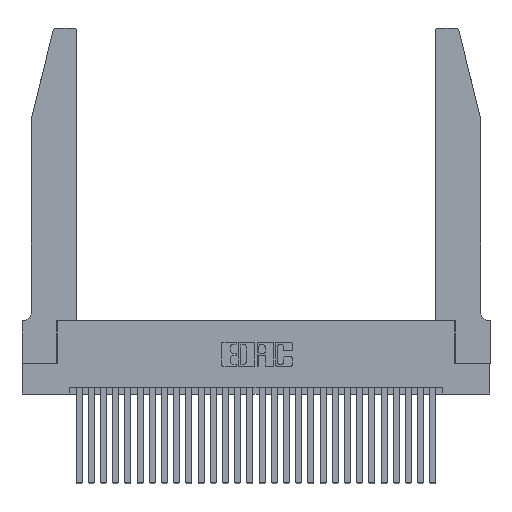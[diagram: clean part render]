
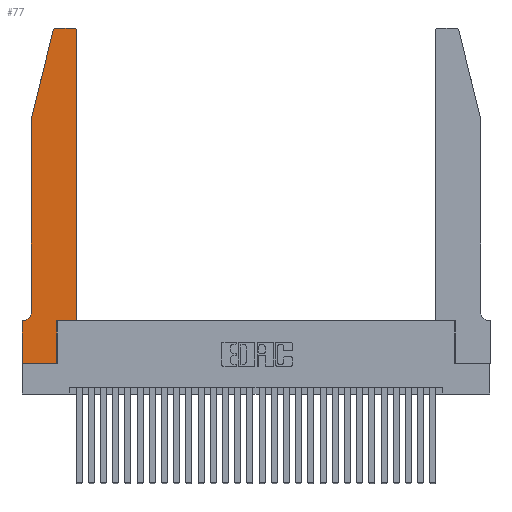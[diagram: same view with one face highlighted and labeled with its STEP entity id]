
A CAD part, top view. The second image highlights one B-rep face of the part: STEP entity #77.
In plain terms, the highlighted planar face has unit normal (0, 0, 1).
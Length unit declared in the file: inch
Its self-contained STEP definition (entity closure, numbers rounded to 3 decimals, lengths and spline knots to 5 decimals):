
#77 = ADVANCED_FACE ( 'NONE', ( #26338 ), #5911, .T. ) ;
#261 = DIRECTION ( 'NONE',  ( -0.239, -0.971, 0. ) ) ;
#552 = DIRECTION ( 'NONE',  ( -1., 0., 0. ) ) ;
#562 = ORIENTED_EDGE ( 'NONE', *, *, #4108, .T. ) ;
#1627 = DIRECTION ( 'NONE',  ( -1., 0., 0. ) ) ;
#1837 = ORIENTED_EDGE ( 'NONE', *, *, #16218, .T. ) ;
#2199 = VECTOR ( 'NONE', #18765, 39.37008 ) ;
#2435 = CARTESIAN_POINT ( 'NONE',  ( 0.284, 2.75, 0.37 ) ) ;
#3099 = DIRECTION ( 'NONE',  ( 0., -1., 0. ) ) ;
#3927 = CARTESIAN_POINT ( 'NONE',  ( 0.4205, 2.75, 0.37 ) ) ;
#4108 = EDGE_CURVE ( 'NONE', #5918, #16222, #10829, .T. ) ;
#5079 = EDGE_CURVE ( 'NONE', #28512, #18662, #29713, .T. ) ;
#5210 = ORIENTED_EDGE ( 'NONE', *, *, #26392, .T. ) ;
#5576 = VECTOR ( 'NONE', #8357, 39.37008 ) ;
#5631 = LINE ( 'NONE', #8975, #16499 ) ;
#5864 = DIRECTION ( 'NONE',  ( 0., 1., 0. ) ) ;
#5896 = VECTOR ( 'NONE', #9201, 39.37008 ) ;
#5911 = PLANE ( 'NONE',  #17791 ) ;
#5918 = VERTEX_POINT ( 'NONE', #26339 ) ;
#6234 = AXIS2_PLACEMENT_3D ( 'NONE', #11985, #27844, #14289 ) ;
#7351 = LINE ( 'NONE', #25167, #5896 ) ;
#8357 = DIRECTION ( 'NONE',  ( 1., 0., 0. ) ) ;
#8621 = EDGE_CURVE ( 'NONE', #22526, #9261, #5631, .T. ) ;
#8630 = CARTESIAN_POINT ( 'NONE',  ( 0., 0.35, 0.37 ) ) ;
#8869 = LINE ( 'NONE', #22281, #13567 ) ;
#8975 = CARTESIAN_POINT ( 'NONE',  ( 0., 0., 0.37 ) ) ;
#9042 = CARTESIAN_POINT ( 'NONE',  ( 0.2865, 0., 0.37 ) ) ;
#9201 = DIRECTION ( 'NONE',  ( 0., -1., 0. ) ) ;
#9261 = VERTEX_POINT ( 'NONE', #9042 ) ;
#9852 = ORIENTED_EDGE ( 'NONE', *, *, #10939, .T. ) ;
#9996 = CARTESIAN_POINT ( 'NONE',  ( 0.2605, 2.75, 0.37 ) ) ;
#10221 = VERTEX_POINT ( 'NONE', #15448 ) ;
#10367 = DIRECTION ( 'NONE',  ( 0., 0., 1. ) ) ;
#10577 = CARTESIAN_POINT ( 'NONE',  ( 0.4505, 0.35, 0.37 ) ) ;
#10829 = CIRCLE ( 'NONE', #6234, 0.03 ) ;
#10939 = EDGE_CURVE ( 'NONE', #20182, #22526, #7351, .T. ) ;
#11081 = EDGE_CURVE ( 'NONE', #12643, #5918, #14593, .T. ) ;
#11454 = VECTOR ( 'NONE', #5864, 39.37008 ) ;
#11659 = CARTESIAN_POINT ( 'NONE',  ( 0., 0., 0.37 ) ) ;
#11985 = CARTESIAN_POINT ( 'NONE',  ( 0.4205, 2.72, 0.37 ) ) ;
#12000 = CIRCLE ( 'NONE', #26807, 0.07 ) ;
#12643 = VERTEX_POINT ( 'NONE', #28993 ) ;
#12751 = ORIENTED_EDGE ( 'NONE', *, *, #15363, .T. ) ;
#13154 = CARTESIAN_POINT ( 'NONE',  ( 0.25487, 2.72718, 0.37 ) ) ;
#13567 = VECTOR ( 'NONE', #29037, 39.37008 ) ;
#14289 = DIRECTION ( 'NONE',  ( 1., 0., 0. ) ) ;
#14382 = CARTESIAN_POINT ( 'NONE',  ( 0.0755, 2., 0.37 ) ) ;
#14593 = LINE ( 'NONE', #16482, #2199 ) ;
#14709 = VECTOR ( 'NONE', #3099, 39.37008 ) ;
#15054 = ORIENTED_EDGE ( 'NONE', *, *, #11081, .T. ) ;
#15118 = CARTESIAN_POINT ( 'NONE',  ( 0.0755, 2., 0.37 ) ) ;
#15363 = EDGE_CURVE ( 'NONE', #16222, #23234, #18998, .T. ) ;
#15448 = CARTESIAN_POINT ( 'NONE',  ( 0.2865, 0.35, 0.37 ) ) ;
#15557 = DIRECTION ( 'NONE',  ( 0., 0., -1. ) ) ;
#16218 = EDGE_CURVE ( 'NONE', #18629, #20182, #8869, .T. ) ;
#16222 = VERTEX_POINT ( 'NONE', #3927 ) ;
#16482 = CARTESIAN_POINT ( 'NONE',  ( 0.4505, 0.35, 0.37 ) ) ;
#16499 = VECTOR ( 'NONE', #29437, 39.37008 ) ;
#16911 = ORIENTED_EDGE ( 'NONE', *, *, #19926, .T. ) ;
#17079 = VECTOR ( 'NONE', #261, 39.37008 ) ;
#17348 = CARTESIAN_POINT ( 'NONE',  ( 0.0055, 0.35, 0.37 ) ) ;
#17791 = AXIS2_PLACEMENT_3D ( 'NONE', #23497, #18524, #18530 ) ;
#17871 = LINE ( 'NONE', #10577, #5576 ) ;
#18524 = DIRECTION ( 'NONE',  ( 0., 0., 1. ) ) ;
#18530 = DIRECTION ( 'NONE',  ( 1., 0., 0. ) ) ;
#18629 = VERTEX_POINT ( 'NONE', #17348 ) ;
#18662 = VERTEX_POINT ( 'NONE', #15118 ) ;
#18765 = DIRECTION ( 'NONE',  ( 0., 1., 0. ) ) ;
#18998 = LINE ( 'NONE', #9996, #29518 ) ;
#19298 = CARTESIAN_POINT ( 'NONE',  ( 0.0755, 2., 0.37 ) ) ;
#19926 = EDGE_CURVE ( 'NONE', #18662, #20373, #20785, .T. ) ;
#20182 = VERTEX_POINT ( 'NONE', #8630 ) ;
#20373 = VERTEX_POINT ( 'NONE', #23029 ) ;
#20785 = LINE ( 'NONE', #19298, #14709 ) ;
#20939 = AXIS2_PLACEMENT_3D ( 'NONE', #24038, #10367, #26295 ) ;
#21569 = ORIENTED_EDGE ( 'NONE', *, *, #8621, .T. ) ;
#21855 = EDGE_CURVE ( 'NONE', #23234, #28512, #29075, .T. ) ;
#22200 = ORIENTED_EDGE ( 'NONE', *, *, #5079, .T. ) ;
#22281 = CARTESIAN_POINT ( 'NONE',  ( 0.0755, 0.35, 0.37 ) ) ;
#22526 = VERTEX_POINT ( 'NONE', #11659 ) ;
#22997 = EDGE_CURVE ( 'NONE', #20373, #18629, #12000, .T. ) ;
#23029 = CARTESIAN_POINT ( 'NONE',  ( 0.0755, 0.42, 0.37 ) ) ;
#23234 = VERTEX_POINT ( 'NONE', #2435 ) ;
#23497 = CARTESIAN_POINT ( 'NONE',  ( 0., 0.35, 0.37 ) ) ;
#24038 = CARTESIAN_POINT ( 'NONE',  ( 0.284, 2.72, 0.37 ) ) ;
#24200 = CARTESIAN_POINT ( 'NONE',  ( 0.2865, 0.35, 0.37 ) ) ;
#24376 = ORIENTED_EDGE ( 'NONE', *, *, #25221, .T. ) ;
#24595 = ORIENTED_EDGE ( 'NONE', *, *, #21855, .T. ) ;
#25167 = CARTESIAN_POINT ( 'NONE',  ( 0., 0., 0.37 ) ) ;
#25221 = EDGE_CURVE ( 'NONE', #9261, #10221, #29521, .T. ) ;
#26295 = DIRECTION ( 'NONE',  ( 1., 0., 0. ) ) ;
#26338 = FACE_OUTER_BOUND ( 'NONE', #28379, .T. ) ;
#26339 = CARTESIAN_POINT ( 'NONE',  ( 0.4505, 2.72, 0.37 ) ) ;
#26392 = EDGE_CURVE ( 'NONE', #10221, #12643, #17871, .T. ) ;
#26807 = AXIS2_PLACEMENT_3D ( 'NONE', #29078, #15557, #1627 ) ;
#26995 = ORIENTED_EDGE ( 'NONE', *, *, #22997, .T. ) ;
#27844 = DIRECTION ( 'NONE',  ( 0., 0., 1. ) ) ;
#28379 = EDGE_LOOP ( 'NONE', ( #12751, #24595, #22200, #16911, #26995, #1837, #9852, #21569, #24376, #5210, #15054, #562 ) ) ;
#28512 = VERTEX_POINT ( 'NONE', #13154 ) ;
#28993 = CARTESIAN_POINT ( 'NONE',  ( 0.4505, 0.35, 0.37 ) ) ;
#29037 = DIRECTION ( 'NONE',  ( -1., 0., 0. ) ) ;
#29075 = CIRCLE ( 'NONE', #20939, 0.03 ) ;
#29078 = CARTESIAN_POINT ( 'NONE',  ( 0.0055, 0.42, 0.37 ) ) ;
#29437 = DIRECTION ( 'NONE',  ( 1., 0., 0. ) ) ;
#29518 = VECTOR ( 'NONE', #552, 39.37008 ) ;
#29521 = LINE ( 'NONE', #24200, #11454 ) ;
#29713 = LINE ( 'NONE', #14382, #17079 ) ;
